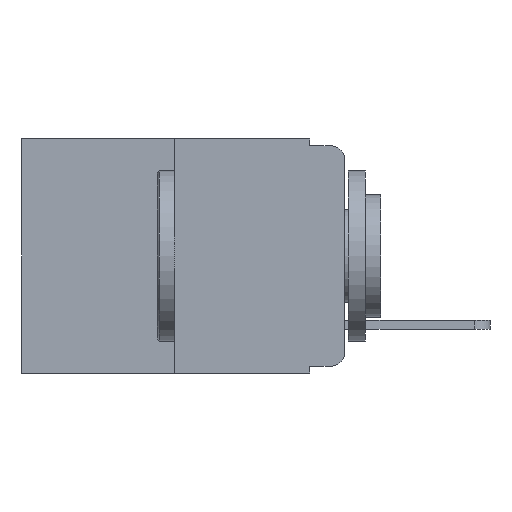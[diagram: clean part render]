
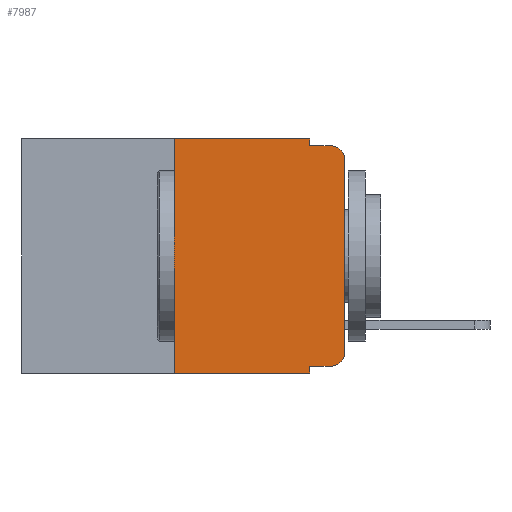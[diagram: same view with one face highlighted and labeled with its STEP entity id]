
A CAD part, left-side view. The second image highlights one B-rep face of the part: STEP entity #7987.
In plain terms, the highlighted planar face has unit normal (-1, 0, 0).
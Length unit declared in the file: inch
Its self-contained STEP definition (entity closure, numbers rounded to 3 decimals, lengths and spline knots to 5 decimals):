
#401 = CARTESIAN_POINT ( 'NONE',  ( 0., 0.051, 0. ) ) ;
#629 = CARTESIAN_POINT ( 'NONE',  ( 0., 0., -0.313 ) ) ;
#1236 = DIRECTION ( 'NONE',  ( 0., -1., 0. ) ) ;
#1881 = LINE ( 'NONE', #8305, #2687 ) ;
#2054 = VERTEX_POINT ( 'NONE', #20985 ) ;
#2136 = CARTESIAN_POINT ( 'NONE',  ( 0., 0.051, -0.333 ) ) ;
#2322 = EDGE_CURVE ( 'NONE', #4083, #9804, #14898, .T. ) ;
#2363 = VERTEX_POINT ( 'NONE', #16261 ) ;
#2615 = DIRECTION ( 'NONE',  ( 0., 0., -1. ) ) ;
#2687 = VECTOR ( 'NONE', #20375, 39.37008 ) ;
#3025 = DIRECTION ( 'NONE',  ( 0., 0., 1. ) ) ;
#3179 = VERTEX_POINT ( 'NONE', #15736 ) ;
#3195 = CARTESIAN_POINT ( 'NONE',  ( 0., 0.051, -0.333 ) ) ;
#3554 = AXIS2_PLACEMENT_3D ( 'NONE', #11679, #13437, #6188 ) ;
#3608 = DIRECTION ( 'NONE',  ( 0., 0., -1. ) ) ;
#3759 = PLANE ( 'NONE',  #18835 ) ;
#4083 = VERTEX_POINT ( 'NONE', #18828 ) ;
#4221 = EDGE_CURVE ( 'NONE', #9804, #7989, #11453, .T. ) ;
#4366 = EDGE_CURVE ( 'NONE', #7032, #3179, #9577, .T. ) ;
#4628 = VECTOR ( 'NONE', #5837, 39.37008 ) ;
#4748 = CARTESIAN_POINT ( 'NONE',  ( 0., 0.051, 0. ) ) ;
#5086 = CARTESIAN_POINT ( 'NONE',  ( 0., 0.051, -0.01 ) ) ;
#5129 = ORIENTED_EDGE ( 'NONE', *, *, #4366, .T. ) ;
#5315 = CARTESIAN_POINT ( 'NONE',  ( 0., 0.473, 0. ) ) ;
#5552 = VECTOR ( 'NONE', #1236, 39.37008 ) ;
#5837 = DIRECTION ( 'NONE',  ( 0., 0., 1. ) ) ;
#6172 = ORIENTED_EDGE ( 'NONE', *, *, #2322, .F. ) ;
#6188 = DIRECTION ( 'NONE',  ( 0., 0., -1. ) ) ;
#6385 = VERTEX_POINT ( 'NONE', #10300 ) ;
#6480 = EDGE_CURVE ( 'NONE', #7032, #2054, #21853, .T. ) ;
#7032 = VERTEX_POINT ( 'NONE', #2136 ) ;
#7567 = DIRECTION ( 'NONE',  ( 0., -1., 0. ) ) ;
#7800 = CARTESIAN_POINT ( 'NONE',  ( 0., 0.25, 0. ) ) ;
#7830 = VECTOR ( 'NONE', #2615, 39.37008 ) ;
#7987 = ADVANCED_FACE ( 'NONE', ( #19908 ), #3759, .F. ) ;
#7989 = VERTEX_POINT ( 'NONE', #5086 ) ;
#8305 = CARTESIAN_POINT ( 'NONE',  ( 0., 0.051, -0.01 ) ) ;
#9114 = AXIS2_PLACEMENT_3D ( 'NONE', #13664, #19014, #13588 ) ;
#9577 = LINE ( 'NONE', #3195, #5552 ) ;
#9751 = EDGE_CURVE ( 'NONE', #6385, #4083, #17171, .T. ) ;
#9804 = VERTEX_POINT ( 'NONE', #401 ) ;
#10300 = CARTESIAN_POINT ( 'NONE',  ( 0., 0.25, -0.343 ) ) ;
#10394 = ORIENTED_EDGE ( 'NONE', *, *, #9751, .F. ) ;
#11317 = DIRECTION ( 'NONE',  ( 0., -1., 0. ) ) ;
#11393 = VERTEX_POINT ( 'NONE', #15911 ) ;
#11453 = LINE ( 'NONE', #4748, #19822 ) ;
#11665 = ORIENTED_EDGE ( 'NONE', *, *, #4221, .F. ) ;
#11679 = CARTESIAN_POINT ( 'NONE',  ( 0., 0.02, -0.313 ) ) ;
#11918 = VECTOR ( 'NONE', #7567, 39.37008 ) ;
#11971 = ORIENTED_EDGE ( 'NONE', *, *, #21422, .T. ) ;
#12895 = CARTESIAN_POINT ( 'NONE',  ( 0., 0.051, 0. ) ) ;
#13304 = VECTOR ( 'NONE', #11317, 39.37008 ) ;
#13437 = DIRECTION ( 'NONE',  ( -1., 0., 0. ) ) ;
#13588 = DIRECTION ( 'NONE',  ( 0., 0., -1. ) ) ;
#13664 = CARTESIAN_POINT ( 'NONE',  ( 0., 0.02, -0.03 ) ) ;
#14898 = LINE ( 'NONE', #17632, #11918 ) ;
#15160 = EDGE_CURVE ( 'NONE', #16312, #2363, #19459, .T. ) ;
#15306 = EDGE_CURVE ( 'NONE', #3179, #16312, #20542, .T. ) ;
#15454 = LINE ( 'NONE', #18348, #13304 ) ;
#15736 = CARTESIAN_POINT ( 'NONE',  ( 0., 0.02, -0.333 ) ) ;
#15911 = CARTESIAN_POINT ( 'NONE',  ( 0., 0.02, -0.01 ) ) ;
#16261 = CARTESIAN_POINT ( 'NONE',  ( 0., 0., -0.03 ) ) ;
#16312 = VERTEX_POINT ( 'NONE', #629 ) ;
#16373 = ORIENTED_EDGE ( 'NONE', *, *, #15306, .T. ) ;
#16925 = EDGE_CURVE ( 'NONE', #7989, #11393, #1881, .T. ) ;
#17171 = LINE ( 'NONE', #7800, #17948 ) ;
#17358 = DIRECTION ( 'NONE',  ( 1., 0., 0. ) ) ;
#17630 = CIRCLE ( 'NONE', #9114, 0.02 ) ;
#17632 = CARTESIAN_POINT ( 'NONE',  ( 0., 0.473, 0. ) ) ;
#17722 = DIRECTION ( 'NONE',  ( 0., 0., -1. ) ) ;
#17948 = VECTOR ( 'NONE', #3025, 39.37008 ) ;
#18020 = ORIENTED_EDGE ( 'NONE', *, *, #21632, .T. ) ;
#18348 = CARTESIAN_POINT ( 'NONE',  ( 0., 0.473, -0.343 ) ) ;
#18536 = EDGE_LOOP ( 'NONE', ( #19464, #18020, #21780, #11665, #6172, #10394, #11971, #19720, #5129, #16373 ) ) ;
#18828 = CARTESIAN_POINT ( 'NONE',  ( 0., 0.25, 0. ) ) ;
#18835 = AXIS2_PLACEMENT_3D ( 'NONE', #5315, #17358, #3608 ) ;
#19014 = DIRECTION ( 'NONE',  ( -1., 0., 0. ) ) ;
#19459 = LINE ( 'NONE', #21635, #4628 ) ;
#19464 = ORIENTED_EDGE ( 'NONE', *, *, #15160, .T. ) ;
#19720 = ORIENTED_EDGE ( 'NONE', *, *, #6480, .F. ) ;
#19822 = VECTOR ( 'NONE', #17722, 39.37008 ) ;
#19908 = FACE_OUTER_BOUND ( 'NONE', #18536, .T. ) ;
#20375 = DIRECTION ( 'NONE',  ( 0., -1., 0. ) ) ;
#20542 = CIRCLE ( 'NONE', #3554, 0.02 ) ;
#20985 = CARTESIAN_POINT ( 'NONE',  ( 0., 0.051, -0.343 ) ) ;
#21422 = EDGE_CURVE ( 'NONE', #6385, #2054, #15454, .T. ) ;
#21632 = EDGE_CURVE ( 'NONE', #2363, #11393, #17630, .T. ) ;
#21635 = CARTESIAN_POINT ( 'NONE',  ( 0., 0., 0. ) ) ;
#21780 = ORIENTED_EDGE ( 'NONE', *, *, #16925, .F. ) ;
#21853 = LINE ( 'NONE', #12895, #7830 ) ;
